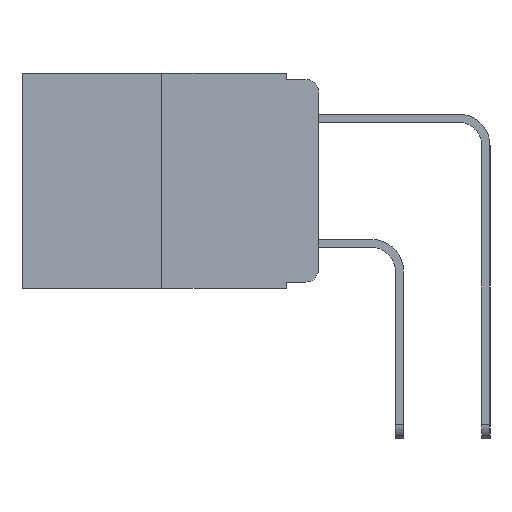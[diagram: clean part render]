
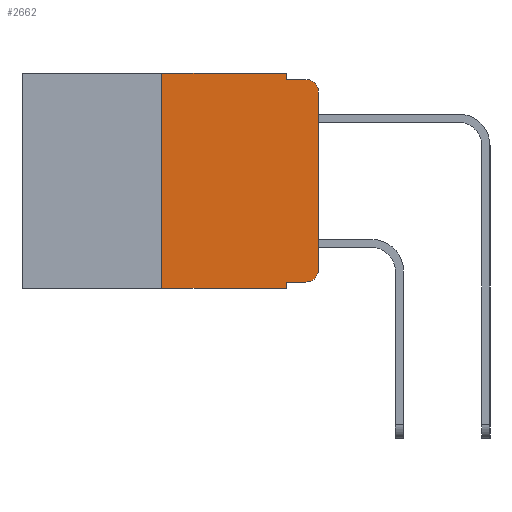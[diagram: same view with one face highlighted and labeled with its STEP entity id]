
A CAD part, left-side view. The second image highlights one B-rep face of the part: STEP entity #2662.
In plain terms, the highlighted planar face has unit normal (-1, 0, 0).
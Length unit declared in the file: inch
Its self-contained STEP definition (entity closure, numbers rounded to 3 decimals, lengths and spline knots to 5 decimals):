
#24 = CARTESIAN_POINT ( 'NONE',  ( 0., 0.473, 0. ) ) ;
#323 = ORIENTED_EDGE ( 'NONE', *, *, #24331, .T. ) ;
#344 = ORIENTED_EDGE ( 'NONE', *, *, #21942, .T. ) ;
#1695 = VERTEX_POINT ( 'NONE', #12191 ) ;
#1748 = CARTESIAN_POINT ( 'NONE',  ( 0., 0., -0.03 ) ) ;
#1889 = DIRECTION ( 'NONE',  ( 1., 0., 0. ) ) ;
#1975 = ORIENTED_EDGE ( 'NONE', *, *, #8740, .F. ) ;
#2137 = DIRECTION ( 'NONE',  ( 0., -1., 0. ) ) ;
#2517 = VERTEX_POINT ( 'NONE', #21996 ) ;
#2624 = ORIENTED_EDGE ( 'NONE', *, *, #15710, .F. ) ;
#2662 = ADVANCED_FACE ( 'NONE', ( #21081 ), #19680, .F. ) ;
#2782 = CARTESIAN_POINT ( 'NONE',  ( 0., 0.051, 0. ) ) ;
#3510 = CARTESIAN_POINT ( 'NONE',  ( 0., 0.25, 0. ) ) ;
#3628 = ORIENTED_EDGE ( 'NONE', *, *, #5450, .T. ) ;
#4086 = DIRECTION ( 'NONE',  ( 0., 0., -1. ) ) ;
#4257 = DIRECTION ( 'NONE',  ( 0., -1., 0. ) ) ;
#4345 = VERTEX_POINT ( 'NONE', #4552 ) ;
#4552 = CARTESIAN_POINT ( 'NONE',  ( 0., 0.02, -0.333 ) ) ;
#4765 = EDGE_CURVE ( 'NONE', #8983, #8538, #9627, .T. ) ;
#5450 = EDGE_CURVE ( 'NONE', #2517, #8538, #23813, .T. ) ;
#6492 = VERTEX_POINT ( 'NONE', #18535 ) ;
#7236 = EDGE_LOOP ( 'NONE', ( #13207, #11336, #9838, #1975, #2624, #24506, #3628, #7395, #323, #344 ) ) ;
#7395 = ORIENTED_EDGE ( 'NONE', *, *, #4765, .F. ) ;
#7416 = EDGE_CURVE ( 'NONE', #2517, #23119, #20074, .T. ) ;
#8538 = VERTEX_POINT ( 'NONE', #14375 ) ;
#8597 = CIRCLE ( 'NONE', #11325, 0.02 ) ;
#8740 = EDGE_CURVE ( 'NONE', #22904, #15185, #18242, .T. ) ;
#8983 = VERTEX_POINT ( 'NONE', #18029 ) ;
#9324 = DIRECTION ( 'NONE',  ( -1., 0., 0. ) ) ;
#9364 = DIRECTION ( 'NONE',  ( 0., -1., 0. ) ) ;
#9627 = LINE ( 'NONE', #11927, #19214 ) ;
#9742 = LINE ( 'NONE', #20780, #15482 ) ;
#9829 = CARTESIAN_POINT ( 'NONE',  ( 0., 0.02, -0.313 ) ) ;
#9838 = ORIENTED_EDGE ( 'NONE', *, *, #10025, .F. ) ;
#10025 = EDGE_CURVE ( 'NONE', #15185, #6492, #9742, .T. ) ;
#10196 = VECTOR ( 'NONE', #4257, 39.37008 ) ;
#11081 = DIRECTION ( 'NONE',  ( 0., 0., -1. ) ) ;
#11325 = AXIS2_PLACEMENT_3D ( 'NONE', #9829, #23031, #11800 ) ;
#11336 = ORIENTED_EDGE ( 'NONE', *, *, #11341, .T. ) ;
#11341 = EDGE_CURVE ( 'NONE', #14563, #6492, #13343, .T. ) ;
#11800 = DIRECTION ( 'NONE',  ( 0., 0., -1. ) ) ;
#11809 = CARTESIAN_POINT ( 'NONE',  ( 0., 0.473, -0.343 ) ) ;
#11850 = DIRECTION ( 'NONE',  ( 0., 0., 1. ) ) ;
#11927 = CARTESIAN_POINT ( 'NONE',  ( 0., 0.051, 0. ) ) ;
#11936 = CARTESIAN_POINT ( 'NONE',  ( 0., 0., 0. ) ) ;
#12191 = CARTESIAN_POINT ( 'NONE',  ( 0., 0., -0.313 ) ) ;
#13184 = VECTOR ( 'NONE', #22772, 39.37008 ) ;
#13207 = ORIENTED_EDGE ( 'NONE', *, *, #17756, .T. ) ;
#13343 = CIRCLE ( 'NONE', #22716, 0.02 ) ;
#13807 = CARTESIAN_POINT ( 'NONE',  ( 0., 0.473, 0. ) ) ;
#13918 = VECTOR ( 'NONE', #23041, 39.37008 ) ;
#13964 = VECTOR ( 'NONE', #11850, 39.37008 ) ;
#14006 = CARTESIAN_POINT ( 'NONE',  ( 0., 0.051, -0.333 ) ) ;
#14375 = CARTESIAN_POINT ( 'NONE',  ( 0., 0.051, -0.343 ) ) ;
#14563 = VERTEX_POINT ( 'NONE', #1748 ) ;
#14609 = CARTESIAN_POINT ( 'NONE',  ( 0., 0.25, 0. ) ) ;
#14618 = AXIS2_PLACEMENT_3D ( 'NONE', #13807, #1889, #11081 ) ;
#15185 = VERTEX_POINT ( 'NONE', #24424 ) ;
#15327 = LINE ( 'NONE', #14006, #10196 ) ;
#15482 = VECTOR ( 'NONE', #9364, 39.37008 ) ;
#15710 = EDGE_CURVE ( 'NONE', #23119, #22904, #22885, .T. ) ;
#16444 = DIRECTION ( 'NONE',  ( 0., 0., 1. ) ) ;
#17756 = EDGE_CURVE ( 'NONE', #1695, #14563, #18442, .T. ) ;
#18029 = CARTESIAN_POINT ( 'NONE',  ( 0., 0.051, -0.333 ) ) ;
#18242 = LINE ( 'NONE', #19022, #13184 ) ;
#18442 = LINE ( 'NONE', #11936, #13964 ) ;
#18535 = CARTESIAN_POINT ( 'NONE',  ( 0., 0.02, -0.01 ) ) ;
#19022 = CARTESIAN_POINT ( 'NONE',  ( 0., 0.051, 0. ) ) ;
#19214 = VECTOR ( 'NONE', #4086, 39.37008 ) ;
#19680 = PLANE ( 'NONE',  #14618 ) ;
#20074 = LINE ( 'NONE', #14609, #24837 ) ;
#20738 = CARTESIAN_POINT ( 'NONE',  ( 0., 0.02, -0.03 ) ) ;
#20780 = CARTESIAN_POINT ( 'NONE',  ( 0., 0.051, -0.01 ) ) ;
#21081 = FACE_OUTER_BOUND ( 'NONE', #7236, .T. ) ;
#21942 = EDGE_CURVE ( 'NONE', #4345, #1695, #8597, .T. ) ;
#21996 = CARTESIAN_POINT ( 'NONE',  ( 0., 0.25, -0.343 ) ) ;
#22327 = VECTOR ( 'NONE', #2137, 39.37008 ) ;
#22545 = DIRECTION ( 'NONE',  ( 0., 0., -1. ) ) ;
#22716 = AXIS2_PLACEMENT_3D ( 'NONE', #20738, #9324, #22545 ) ;
#22772 = DIRECTION ( 'NONE',  ( 0., 0., -1. ) ) ;
#22885 = LINE ( 'NONE', #24, #22327 ) ;
#22904 = VERTEX_POINT ( 'NONE', #2782 ) ;
#23031 = DIRECTION ( 'NONE',  ( -1., 0., 0. ) ) ;
#23041 = DIRECTION ( 'NONE',  ( 0., -1., 0. ) ) ;
#23119 = VERTEX_POINT ( 'NONE', #3510 ) ;
#23813 = LINE ( 'NONE', #11809, #13918 ) ;
#24331 = EDGE_CURVE ( 'NONE', #8983, #4345, #15327, .T. ) ;
#24424 = CARTESIAN_POINT ( 'NONE',  ( 0., 0.051, -0.01 ) ) ;
#24506 = ORIENTED_EDGE ( 'NONE', *, *, #7416, .F. ) ;
#24837 = VECTOR ( 'NONE', #16444, 39.37008 ) ;
